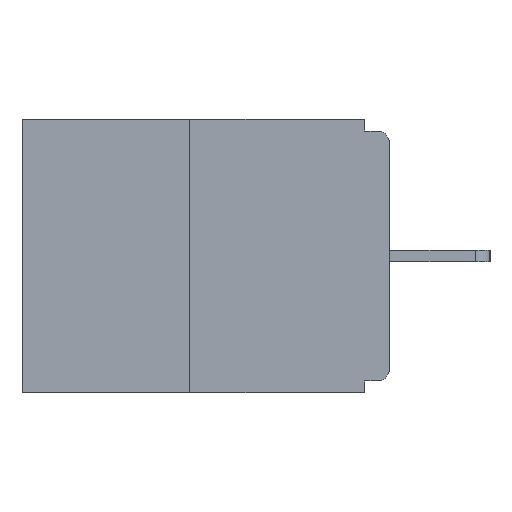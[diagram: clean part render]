
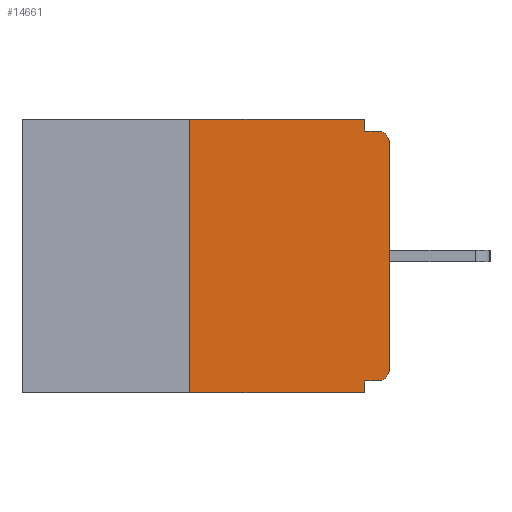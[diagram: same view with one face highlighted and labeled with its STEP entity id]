
A CAD part, left-side view. The second image highlights one B-rep face of the part: STEP entity #14661.
In plain terms, the highlighted planar face has unit normal (-1, 0, 0).
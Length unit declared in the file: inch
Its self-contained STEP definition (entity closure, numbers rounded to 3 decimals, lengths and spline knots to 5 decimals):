
#162 = ORIENTED_EDGE ( 'NONE', *, *, #7193, .T. ) ;
#311 = EDGE_CURVE ( 'NONE', #10781, #15480, #18579, .T. ) ;
#1272 = ORIENTED_EDGE ( 'NONE', *, *, #311, .T. ) ;
#1392 = ORIENTED_EDGE ( 'NONE', *, *, #20341, .F. ) ;
#2023 = CARTESIAN_POINT ( 'NONE',  ( 0., 0.46, -0.343 ) ) ;
#2104 = VERTEX_POINT ( 'NONE', #18230 ) ;
#2542 = VERTEX_POINT ( 'NONE', #16322 ) ;
#2794 = EDGE_CURVE ( 'NONE', #19755, #8220, #4882, .T. ) ;
#2848 = CARTESIAN_POINT ( 'NONE',  ( 0., 0.015, -0.03 ) ) ;
#2915 = EDGE_CURVE ( 'NONE', #8220, #2104, #16796, .T. ) ;
#2942 = ORIENTED_EDGE ( 'NONE', *, *, #17327, .F. ) ;
#3639 = DIRECTION ( 'NONE',  ( -1., 0., 0. ) ) ;
#3668 = CARTESIAN_POINT ( 'NONE',  ( 0., 0., 0. ) ) ;
#4702 = EDGE_CURVE ( 'NONE', #2542, #17175, #10190, .T. ) ;
#4882 = LINE ( 'NONE', #5089, #12874 ) ;
#5089 = CARTESIAN_POINT ( 'NONE',  ( 0., 0.031, 0. ) ) ;
#5223 = AXIS2_PLACEMENT_3D ( 'NONE', #17958, #3639, #8857 ) ;
#5260 = ORIENTED_EDGE ( 'NONE', *, *, #4702, .T. ) ;
#5403 = EDGE_LOOP ( 'NONE', ( #2942, #9242, #5260, #1392, #12201, #1272, #14247, #162, #5810, #17382 ) ) ;
#5697 = DIRECTION ( 'NONE',  ( 0., -1., 0. ) ) ;
#5810 = ORIENTED_EDGE ( 'NONE', *, *, #2915, .F. ) ;
#5887 = VECTOR ( 'NONE', #11879, 39.37008 ) ;
#6043 = VECTOR ( 'NONE', #17152, 39.37008 ) ;
#6417 = CARTESIAN_POINT ( 'NONE',  ( 0., 0.031, -0.343 ) ) ;
#6553 = CARTESIAN_POINT ( 'NONE',  ( 0., 0.25, 0. ) ) ;
#6615 = LINE ( 'NONE', #16432, #10508 ) ;
#6941 = CARTESIAN_POINT ( 'NONE',  ( 0., 0.46, 0. ) ) ;
#7193 = EDGE_CURVE ( 'NONE', #12642, #2104, #16406, .T. ) ;
#7737 = LINE ( 'NONE', #14127, #6043 ) ;
#8220 = VERTEX_POINT ( 'NONE', #17725 ) ;
#8842 = FACE_OUTER_BOUND ( 'NONE', #5403, .T. ) ;
#8857 = DIRECTION ( 'NONE',  ( 0., 0., -1. ) ) ;
#9103 = VECTOR ( 'NONE', #13312, 39.37008 ) ;
#9242 = ORIENTED_EDGE ( 'NONE', *, *, #16603, .F. ) ;
#9455 = CARTESIAN_POINT ( 'NONE',  ( 0., 0.015, -0.328 ) ) ;
#9706 = DIRECTION ( 'NONE',  ( 0., 1., 0. ) ) ;
#10190 = LINE ( 'NONE', #2023, #13947 ) ;
#10508 = VECTOR ( 'NONE', #12991, 39.37008 ) ;
#10600 = VECTOR ( 'NONE', #18089, 39.37008 ) ;
#10615 = DIRECTION ( 'NONE',  ( 0., 0., -1. ) ) ;
#10638 = CARTESIAN_POINT ( 'NONE',  ( 0., 0., -0.313 ) ) ;
#10781 = VERTEX_POINT ( 'NONE', #9455 ) ;
#11003 = CARTESIAN_POINT ( 'NONE',  ( 0., 0.031, -0.328 ) ) ;
#11713 = LINE ( 'NONE', #3668, #10600 ) ;
#11879 = DIRECTION ( 'NONE',  ( 0., -1., 0. ) ) ;
#12193 = CARTESIAN_POINT ( 'NONE',  ( 0., 0.46, 0. ) ) ;
#12201 = ORIENTED_EDGE ( 'NONE', *, *, #19236, .F. ) ;
#12475 = DIRECTION ( 'NONE',  ( 0., 0., -1. ) ) ;
#12642 = VERTEX_POINT ( 'NONE', #16645 ) ;
#12874 = VECTOR ( 'NONE', #17421, 39.37008 ) ;
#12991 = DIRECTION ( 'NONE',  ( 0., 0., 1. ) ) ;
#13312 = DIRECTION ( 'NONE',  ( 0., -1., 0. ) ) ;
#13419 = LINE ( 'NONE', #6941, #9103 ) ;
#13871 = EDGE_CURVE ( 'NONE', #15480, #12642, #11713, .T. ) ;
#13947 = VECTOR ( 'NONE', #5697, 39.37008 ) ;
#14127 = CARTESIAN_POINT ( 'NONE',  ( 0., 0.031, -0.343 ) ) ;
#14247 = ORIENTED_EDGE ( 'NONE', *, *, #13871, .T. ) ;
#14372 = VERTEX_POINT ( 'NONE', #6553 ) ;
#14661 = ADVANCED_FACE ( 'NONE', ( #8842 ), #17094, .F. ) ;
#15480 = VERTEX_POINT ( 'NONE', #10638 ) ;
#15990 = LINE ( 'NONE', #17447, #18697 ) ;
#16275 = CARTESIAN_POINT ( 'NONE',  ( 0., 0.031, 0. ) ) ;
#16322 = CARTESIAN_POINT ( 'NONE',  ( 0., 0.25, -0.343 ) ) ;
#16406 = CIRCLE ( 'NONE', #17082, 0.015 ) ;
#16432 = CARTESIAN_POINT ( 'NONE',  ( 0., 0.25, 0. ) ) ;
#16603 = EDGE_CURVE ( 'NONE', #2542, #14372, #6615, .T. ) ;
#16645 = CARTESIAN_POINT ( 'NONE',  ( 0., 0., -0.03 ) ) ;
#16796 = LINE ( 'NONE', #19824, #5887 ) ;
#16977 = VERTEX_POINT ( 'NONE', #11003 ) ;
#17082 = AXIS2_PLACEMENT_3D ( 'NONE', #2848, #19248, #12475 ) ;
#17094 = PLANE ( 'NONE',  #20204 ) ;
#17152 = DIRECTION ( 'NONE',  ( 0., 0., -1. ) ) ;
#17175 = VERTEX_POINT ( 'NONE', #6417 ) ;
#17327 = EDGE_CURVE ( 'NONE', #14372, #19755, #13419, .T. ) ;
#17382 = ORIENTED_EDGE ( 'NONE', *, *, #2794, .F. ) ;
#17421 = DIRECTION ( 'NONE',  ( 0., 0., -1. ) ) ;
#17447 = CARTESIAN_POINT ( 'NONE',  ( 0., 0., -0.328 ) ) ;
#17725 = CARTESIAN_POINT ( 'NONE',  ( 0., 0.031, -0.015 ) ) ;
#17958 = CARTESIAN_POINT ( 'NONE',  ( 0., 0.015, -0.313 ) ) ;
#18089 = DIRECTION ( 'NONE',  ( 0., 0., 1. ) ) ;
#18230 = CARTESIAN_POINT ( 'NONE',  ( 0., 0.015, -0.015 ) ) ;
#18564 = DIRECTION ( 'NONE',  ( 1., 0., 0. ) ) ;
#18579 = CIRCLE ( 'NONE', #5223, 0.015 ) ;
#18697 = VECTOR ( 'NONE', #9706, 39.37008 ) ;
#19236 = EDGE_CURVE ( 'NONE', #10781, #16977, #15990, .T. ) ;
#19248 = DIRECTION ( 'NONE',  ( -1., 0., 0. ) ) ;
#19755 = VERTEX_POINT ( 'NONE', #16275 ) ;
#19824 = CARTESIAN_POINT ( 'NONE',  ( 0., 0., -0.015 ) ) ;
#20204 = AXIS2_PLACEMENT_3D ( 'NONE', #12193, #18564, #10615 ) ;
#20341 = EDGE_CURVE ( 'NONE', #16977, #17175, #7737, .T. ) ;
